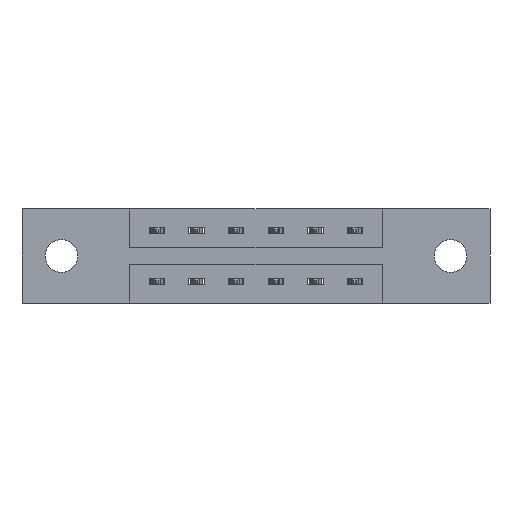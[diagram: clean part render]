
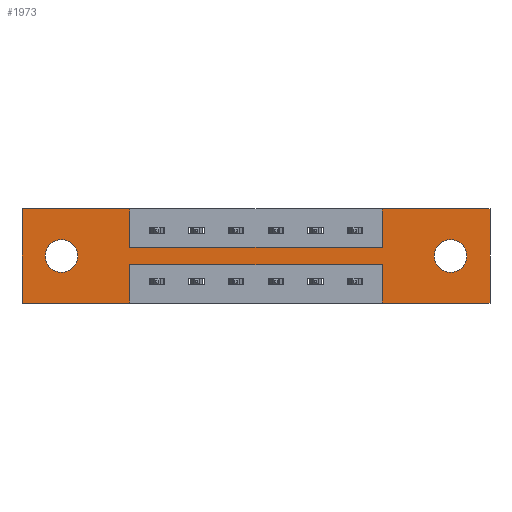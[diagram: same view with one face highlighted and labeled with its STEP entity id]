
A CAD part, front view. The second image highlights one B-rep face of the part: STEP entity #1973.
In plain terms, the highlighted planar face has unit normal (0, -1, 0).
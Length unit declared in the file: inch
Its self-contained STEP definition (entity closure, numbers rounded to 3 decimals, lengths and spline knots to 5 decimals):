
#79 = VERTEX_POINT ( 'NONE', #6029 ) ;
#123 = ORIENTED_EDGE ( 'NONE', *, *, #8577, .F. ) ;
#322 = LINE ( 'NONE', #2010, #7737 ) ;
#355 = ORIENTED_EDGE ( 'NONE', *, *, #8254, .F. ) ;
#485 = VECTOR ( 'NONE', #1804, 39.37008 ) ;
#492 = EDGE_CURVE ( 'NONE', #5400, #2385, #6991, .T. ) ;
#517 = FACE_BOUND ( 'NONE', #2918, .T. ) ;
#532 = LINE ( 'NONE', #6975, #1217 ) ;
#593 = DIRECTION ( 'NONE',  ( -1., 0., 0. ) ) ;
#676 = VERTEX_POINT ( 'NONE', #4305 ) ;
#696 = DIRECTION ( 'NONE',  ( 0., 1., 0. ) ) ;
#703 = ORIENTED_EDGE ( 'NONE', *, *, #5723, .F. ) ;
#708 = VECTOR ( 'NONE', #2479, 39.37008 ) ;
#756 = CARTESIAN_POINT ( 'NONE',  ( 1.417, 0., -0.37 ) ) ;
#760 = CIRCLE ( 'NONE', #6273, 0.064 ) ;
#775 = CARTESIAN_POINT ( 'NONE',  ( 0.425, 0., 0. ) ) ;
#776 = VERTEX_POINT ( 'NONE', #4688 ) ;
#789 = ORIENTED_EDGE ( 'NONE', *, *, #6579, .F. ) ;
#844 = CARTESIAN_POINT ( 'NONE',  ( 1.842, 0., 0. ) ) ;
#891 = VECTOR ( 'NONE', #2208, 39.37008 ) ;
#926 = DIRECTION ( 'NONE',  ( 0., 0., 1. ) ) ;
#956 = DIRECTION ( 'NONE',  ( 1., 0., 0. ) ) ;
#1066 = VECTOR ( 'NONE', #956, 39.37008 ) ;
#1153 = CARTESIAN_POINT ( 'NONE',  ( 1.687, 0., -0.121 ) ) ;
#1164 = VERTEX_POINT ( 'NONE', #8654 ) ;
#1217 = VECTOR ( 'NONE', #593, 39.37008 ) ;
#1308 = VECTOR ( 'NONE', #7372, 39.37008 ) ;
#1439 = ORIENTED_EDGE ( 'NONE', *, *, #7845, .F. ) ;
#1487 = CARTESIAN_POINT ( 'NONE',  ( 0.155, 0., -0.185 ) ) ;
#1530 = FACE_BOUND ( 'NONE', #7427, .T. ) ;
#1578 = VERTEX_POINT ( 'NONE', #8727 ) ;
#1611 = VECTOR ( 'NONE', #6980, 39.37008 ) ;
#1623 = VERTEX_POINT ( 'NONE', #844 ) ;
#1661 = CARTESIAN_POINT ( 'NONE',  ( 1.687, 0., -0.249 ) ) ;
#1662 = CARTESIAN_POINT ( 'NONE',  ( 1.842, 0., -0.37 ) ) ;
#1666 = CARTESIAN_POINT ( 'NONE',  ( 0.425, 0., -0.15 ) ) ;
#1737 = CARTESIAN_POINT ( 'NONE',  ( 1.687, 0., -0.185 ) ) ;
#1739 = EDGE_CURVE ( 'NONE', #2385, #5400, #1982, .T. ) ;
#1804 = DIRECTION ( 'NONE',  ( 1., 0., 0. ) ) ;
#1973 = ADVANCED_FACE ( 'NONE', ( #517, #1530, #8964 ), #3563, .T. ) ;
#1975 = EDGE_LOOP ( 'NONE', ( #8559, #1439, #355, #3055, #123, #6878, #703, #5376, #4840, #9103, #7215, #789 ) ) ;
#1982 = CIRCLE ( 'NONE', #4412, 0.064 ) ;
#2010 = CARTESIAN_POINT ( 'NONE',  ( 0., 0., -0.37 ) ) ;
#2054 = CARTESIAN_POINT ( 'NONE',  ( 1.417, 0., -0.22 ) ) ;
#2055 = CARTESIAN_POINT ( 'NONE',  ( 0., 0., 0. ) ) ;
#2167 = CARTESIAN_POINT ( 'NONE',  ( 0.425, 0., -0.22 ) ) ;
#2169 = VERTEX_POINT ( 'NONE', #1662 ) ;
#2208 = DIRECTION ( 'NONE',  ( 0., 0., 1. ) ) ;
#2268 = LINE ( 'NONE', #7235, #6414 ) ;
#2385 = VERTEX_POINT ( 'NONE', #1153 ) ;
#2390 = LINE ( 'NONE', #8648, #5083 ) ;
#2446 = DIRECTION ( 'NONE',  ( 0., 1., 0. ) ) ;
#2477 = VERTEX_POINT ( 'NONE', #2055 ) ;
#2479 = DIRECTION ( 'NONE',  ( 0., 0., 1. ) ) ;
#2605 = VERTEX_POINT ( 'NONE', #775 ) ;
#2657 = DIRECTION ( 'NONE',  ( 0., 0., -1. ) ) ;
#2799 = EDGE_CURVE ( 'NONE', #2477, #2605, #6012, .T. ) ;
#2833 = AXIS2_PLACEMENT_3D ( 'NONE', #5227, #8825, #926 ) ;
#2893 = ORIENTED_EDGE ( 'NONE', *, *, #492, .T. ) ;
#2918 = EDGE_LOOP ( 'NONE', ( #7709, #2893 ) ) ;
#2930 = DIRECTION ( 'NONE',  ( 0., 1., 0. ) ) ;
#2960 = CARTESIAN_POINT ( 'NONE',  ( 1.417, 0., 0. ) ) ;
#3055 = ORIENTED_EDGE ( 'NONE', *, *, #6632, .F. ) ;
#3218 = LINE ( 'NONE', #1666, #1308 ) ;
#3244 = CARTESIAN_POINT ( 'NONE',  ( 0., 0., 0. ) ) ;
#3477 = CARTESIAN_POINT ( 'NONE',  ( 0., 0., -0.37 ) ) ;
#3563 = PLANE ( 'NONE',  #8269 ) ;
#3801 = VECTOR ( 'NONE', #9087, 39.37008 ) ;
#3909 = DIRECTION ( 'NONE',  ( -1., 0., 0. ) ) ;
#4058 = CARTESIAN_POINT ( 'NONE',  ( 0.425, 0., -0.37 ) ) ;
#4070 = EDGE_CURVE ( 'NONE', #6763, #2477, #2268, .T. ) ;
#4112 = EDGE_CURVE ( 'NONE', #2605, #1578, #2390, .T. ) ;
#4305 = CARTESIAN_POINT ( 'NONE',  ( 1.417, 0., -0.15 ) ) ;
#4412 = AXIS2_PLACEMENT_3D ( 'NONE', #1737, #2446, #5275 ) ;
#4634 = VERTEX_POINT ( 'NONE', #2167 ) ;
#4688 = CARTESIAN_POINT ( 'NONE',  ( 1.417, 0., 0. ) ) ;
#4705 = LINE ( 'NONE', #4058, #3801 ) ;
#4721 = ORIENTED_EDGE ( 'NONE', *, *, #7803, .T. ) ;
#4840 = ORIENTED_EDGE ( 'NONE', *, *, #4112, .F. ) ;
#5067 = DIRECTION ( 'NONE',  ( 0., 0., -1. ) ) ;
#5083 = VECTOR ( 'NONE', #5067, 39.37008 ) ;
#5094 = LINE ( 'NONE', #3244, #485 ) ;
#5227 = CARTESIAN_POINT ( 'NONE',  ( 0.155, 0., -0.185 ) ) ;
#5275 = DIRECTION ( 'NONE',  ( 0., 0., -1. ) ) ;
#5283 = VERTEX_POINT ( 'NONE', #6415 ) ;
#5376 = ORIENTED_EDGE ( 'NONE', *, *, #7005, .F. ) ;
#5400 = VERTEX_POINT ( 'NONE', #1661 ) ;
#5517 = VERTEX_POINT ( 'NONE', #2054 ) ;
#5523 = CARTESIAN_POINT ( 'NONE',  ( 1.842, 0., 0. ) ) ;
#5679 = DIRECTION ( 'NONE',  ( 0., 0., -1. ) ) ;
#5695 = CARTESIAN_POINT ( 'NONE',  ( 0., 0., -0.37 ) ) ;
#5710 = CARTESIAN_POINT ( 'NONE',  ( 1.687, 0., -0.185 ) ) ;
#5723 = EDGE_CURVE ( 'NONE', #676, #776, #8524, .T. ) ;
#5770 = VECTOR ( 'NONE', #3909, 39.37008 ) ;
#6001 = LINE ( 'NONE', #6062, #708 ) ;
#6012 = LINE ( 'NONE', #7388, #1066 ) ;
#6029 = CARTESIAN_POINT ( 'NONE',  ( 0.155, 0., -0.249 ) ) ;
#6061 = EDGE_CURVE ( 'NONE', #4634, #5283, #4705, .T. ) ;
#6062 = CARTESIAN_POINT ( 'NONE',  ( 1.417, 0., -0.37 ) ) ;
#6208 = LINE ( 'NONE', #5523, #1611 ) ;
#6273 = AXIS2_PLACEMENT_3D ( 'NONE', #1487, #2930, #7908 ) ;
#6383 = VERTEX_POINT ( 'NONE', #756 ) ;
#6402 = EDGE_CURVE ( 'NONE', #1164, #79, #760, .T. ) ;
#6414 = VECTOR ( 'NONE', #8037, 39.37008 ) ;
#6415 = CARTESIAN_POINT ( 'NONE',  ( 0.425, 0., -0.37 ) ) ;
#6449 = DIRECTION ( 'NONE',  ( 0., -1., 0. ) ) ;
#6579 = EDGE_CURVE ( 'NONE', #5283, #6763, #532, .T. ) ;
#6632 = EDGE_CURVE ( 'NONE', #2169, #6383, #322, .T. ) ;
#6763 = VERTEX_POINT ( 'NONE', #3477 ) ;
#6800 = CIRCLE ( 'NONE', #2833, 0.064 ) ;
#6878 = ORIENTED_EDGE ( 'NONE', *, *, #8504, .F. ) ;
#6975 = CARTESIAN_POINT ( 'NONE',  ( 0., 0., -0.37 ) ) ;
#6980 = DIRECTION ( 'NONE',  ( 0., 0., -1. ) ) ;
#6991 = CIRCLE ( 'NONE', #8490, 0.064 ) ;
#7005 = EDGE_CURVE ( 'NONE', #1578, #676, #3218, .T. ) ;
#7215 = ORIENTED_EDGE ( 'NONE', *, *, #4070, .F. ) ;
#7235 = CARTESIAN_POINT ( 'NONE',  ( 0., 0., 0. ) ) ;
#7372 = DIRECTION ( 'NONE',  ( 1., 0., 0. ) ) ;
#7388 = CARTESIAN_POINT ( 'NONE',  ( 0., 0., 0. ) ) ;
#7427 = EDGE_LOOP ( 'NONE', ( #9200, #4721 ) ) ;
#7635 = DIRECTION ( 'NONE',  ( -1., 0., 0. ) ) ;
#7709 = ORIENTED_EDGE ( 'NONE', *, *, #1739, .T. ) ;
#7737 = VECTOR ( 'NONE', #7635, 39.37008 ) ;
#7803 = EDGE_CURVE ( 'NONE', #79, #1164, #6800, .T. ) ;
#7845 = EDGE_CURVE ( 'NONE', #5517, #4634, #8256, .T. ) ;
#7908 = DIRECTION ( 'NONE',  ( 0., 0., 1. ) ) ;
#8037 = DIRECTION ( 'NONE',  ( 0., 0., 1. ) ) ;
#8254 = EDGE_CURVE ( 'NONE', #6383, #5517, #6001, .T. ) ;
#8256 = LINE ( 'NONE', #8274, #5770 ) ;
#8269 = AXIS2_PLACEMENT_3D ( 'NONE', #5695, #6449, #2657 ) ;
#8274 = CARTESIAN_POINT ( 'NONE',  ( 0.425, 0., -0.22 ) ) ;
#8490 = AXIS2_PLACEMENT_3D ( 'NONE', #5710, #696, #5679 ) ;
#8504 = EDGE_CURVE ( 'NONE', #776, #1623, #5094, .T. ) ;
#8524 = LINE ( 'NONE', #2960, #891 ) ;
#8559 = ORIENTED_EDGE ( 'NONE', *, *, #6061, .F. ) ;
#8577 = EDGE_CURVE ( 'NONE', #1623, #2169, #6208, .T. ) ;
#8648 = CARTESIAN_POINT ( 'NONE',  ( 0.425, 0., 0. ) ) ;
#8654 = CARTESIAN_POINT ( 'NONE',  ( 0.155, 0., -0.121 ) ) ;
#8727 = CARTESIAN_POINT ( 'NONE',  ( 0.425, 0., -0.15 ) ) ;
#8825 = DIRECTION ( 'NONE',  ( 0., 1., 0. ) ) ;
#8964 = FACE_OUTER_BOUND ( 'NONE', #1975, .T. ) ;
#9087 = DIRECTION ( 'NONE',  ( 0., 0., -1. ) ) ;
#9103 = ORIENTED_EDGE ( 'NONE', *, *, #2799, .F. ) ;
#9200 = ORIENTED_EDGE ( 'NONE', *, *, #6402, .T. ) ;
